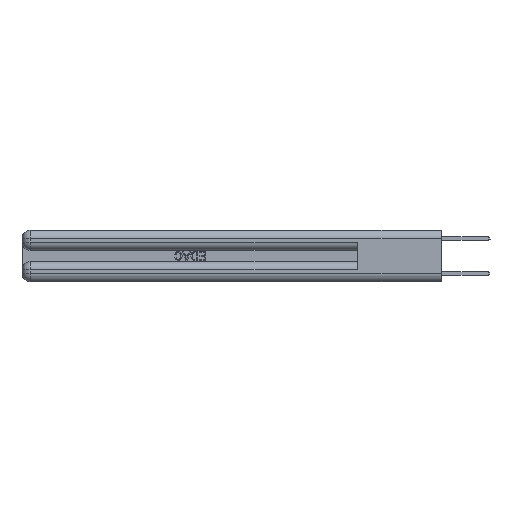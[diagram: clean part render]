
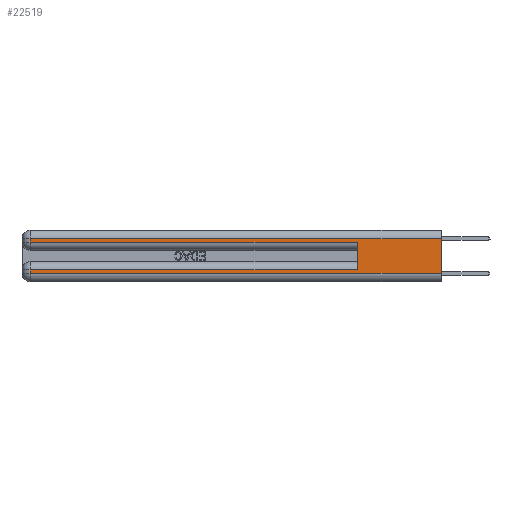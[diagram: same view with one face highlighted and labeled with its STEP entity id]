
A CAD part, left-side view. The second image highlights one B-rep face of the part: STEP entity #22519.
In plain terms, the highlighted planar face has unit normal (-1, 0, 0).
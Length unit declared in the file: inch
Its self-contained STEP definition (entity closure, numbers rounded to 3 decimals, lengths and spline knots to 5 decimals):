
#1219 = CARTESIAN_POINT ( 'NONE',  ( 0., 2.94, 0.31 ) ) ;
#1268 = EDGE_CURVE ( 'NONE', #13163, #10742, #14845, .T. ) ;
#2334 = CARTESIAN_POINT ( 'NONE',  ( 0., 0., 0.37 ) ) ;
#2546 = DIRECTION ( 'NONE',  ( 0., -1., 0. ) ) ;
#2710 = CARTESIAN_POINT ( 'NONE',  ( 0., 2.94, 0.06 ) ) ;
#2910 = ORIENTED_EDGE ( 'NONE', *, *, #23657, .T. ) ;
#2936 = VECTOR ( 'NONE', #23908, 39.37008 ) ;
#3224 = DIRECTION ( 'NONE',  ( 0., -1., 0. ) ) ;
#3884 = CARTESIAN_POINT ( 'NONE',  ( 0., 2.94, 0.37 ) ) ;
#4002 = LINE ( 'NONE', #12608, #23977 ) ;
#4715 = VECTOR ( 'NONE', #18473, 39.37008 ) ;
#4870 = VERTEX_POINT ( 'NONE', #5055 ) ;
#5055 = CARTESIAN_POINT ( 'NONE',  ( 0., 0., 0.31 ) ) ;
#5071 = VERTEX_POINT ( 'NONE', #17904 ) ;
#5363 = CARTESIAN_POINT ( 'NONE',  ( 0., 0.6, 0.085 ) ) ;
#5367 = CARTESIAN_POINT ( 'NONE',  ( 0., 0., 0.06 ) ) ;
#6038 = ORIENTED_EDGE ( 'NONE', *, *, #22864, .F. ) ;
#6070 = EDGE_CURVE ( 'NONE', #21602, #20142, #24003, .T. ) ;
#6347 = DIRECTION ( 'NONE',  ( 0., 0., -1. ) ) ;
#6469 = EDGE_CURVE ( 'NONE', #27179, #5071, #16285, .T. ) ;
#6676 = EDGE_CURVE ( 'NONE', #4870, #27179, #22448, .T. ) ;
#6916 = CARTESIAN_POINT ( 'NONE',  ( 0., 0., 0.31 ) ) ;
#7540 = EDGE_CURVE ( 'NONE', #4870, #10742, #12963, .T. ) ;
#10742 = VERTEX_POINT ( 'NONE', #5367 ) ;
#11629 = VECTOR ( 'NONE', #20229, 39.37008 ) ;
#12608 = CARTESIAN_POINT ( 'NONE',  ( 0., 0.6, 0.145 ) ) ;
#12963 = LINE ( 'NONE', #2334, #25654 ) ;
#13108 = ORIENTED_EDGE ( 'NONE', *, *, #6469, .T. ) ;
#13163 = VERTEX_POINT ( 'NONE', #2710 ) ;
#13819 = CARTESIAN_POINT ( 'NONE',  ( 0., 2.94, 0.085 ) ) ;
#14561 = EDGE_LOOP ( 'NONE', ( #15695, #17423, #13108, #2910, #6038, #26298, #24352, #22345 ) ) ;
#14581 = CARTESIAN_POINT ( 'NONE',  ( 0., 0., 0.085 ) ) ;
#14710 = CARTESIAN_POINT ( 'NONE',  ( 0., 0., 0.285 ) ) ;
#14845 = LINE ( 'NONE', #25678, #23189 ) ;
#15609 = PLANE ( 'NONE',  #25693 ) ;
#15695 = ORIENTED_EDGE ( 'NONE', *, *, #7540, .F. ) ;
#15861 = VECTOR ( 'NONE', #6347, 39.37008 ) ;
#15959 = LINE ( 'NONE', #14710, #28235 ) ;
#16285 = LINE ( 'NONE', #22881, #11629 ) ;
#17423 = ORIENTED_EDGE ( 'NONE', *, *, #6676, .T. ) ;
#17904 = CARTESIAN_POINT ( 'NONE',  ( 0., 2.94, 0.285 ) ) ;
#18473 = DIRECTION ( 'NONE',  ( 0., 1., 0. ) ) ;
#19367 = CARTESIAN_POINT ( 'NONE',  ( 0., 0.6, 0.285 ) ) ;
#20023 = FACE_OUTER_BOUND ( 'NONE', #14561, .T. ) ;
#20142 = VERTEX_POINT ( 'NONE', #13819 ) ;
#20229 = DIRECTION ( 'NONE',  ( 0., 0., -1. ) ) ;
#20747 = DIRECTION ( 'NONE',  ( 0., 0., -1. ) ) ;
#21602 = VERTEX_POINT ( 'NONE', #5363 ) ;
#22345 = ORIENTED_EDGE ( 'NONE', *, *, #1268, .T. ) ;
#22448 = LINE ( 'NONE', #6916, #4715 ) ;
#22519 = ADVANCED_FACE ( 'NONE', ( #20023 ), #15609, .F. ) ;
#22864 = EDGE_CURVE ( 'NONE', #21602, #27749, #4002, .T. ) ;
#22881 = CARTESIAN_POINT ( 'NONE',  ( 0., 2.94, 0.37 ) ) ;
#22889 = DIRECTION ( 'NONE',  ( 0., 0., -1. ) ) ;
#23189 = VECTOR ( 'NONE', #2546, 39.37008 ) ;
#23657 = EDGE_CURVE ( 'NONE', #5071, #27749, #15959, .T. ) ;
#23831 = LINE ( 'NONE', #3884, #15861 ) ;
#23908 = DIRECTION ( 'NONE',  ( 0., 1., 0. ) ) ;
#23977 = VECTOR ( 'NONE', #24065, 39.37008 ) ;
#24003 = LINE ( 'NONE', #14581, #2936 ) ;
#24065 = DIRECTION ( 'NONE',  ( 0., 0., 1. ) ) ;
#24352 = ORIENTED_EDGE ( 'NONE', *, *, #25408, .T. ) ;
#25408 = EDGE_CURVE ( 'NONE', #20142, #13163, #23831, .T. ) ;
#25481 = CARTESIAN_POINT ( 'NONE',  ( 0., 0., 0.37 ) ) ;
#25654 = VECTOR ( 'NONE', #22889, 39.37008 ) ;
#25678 = CARTESIAN_POINT ( 'NONE',  ( 0., 0., 0.06 ) ) ;
#25693 = AXIS2_PLACEMENT_3D ( 'NONE', #25481, #29812, #20747 ) ;
#26298 = ORIENTED_EDGE ( 'NONE', *, *, #6070, .T. ) ;
#27179 = VERTEX_POINT ( 'NONE', #1219 ) ;
#27749 = VERTEX_POINT ( 'NONE', #19367 ) ;
#28235 = VECTOR ( 'NONE', #3224, 39.37008 ) ;
#29812 = DIRECTION ( 'NONE',  ( 1., 0., 0. ) ) ;
